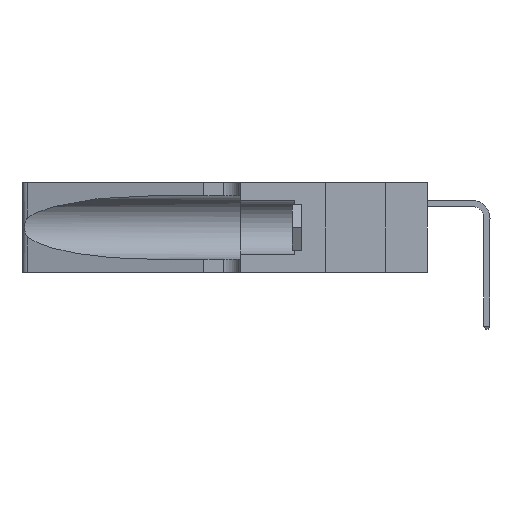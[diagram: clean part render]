
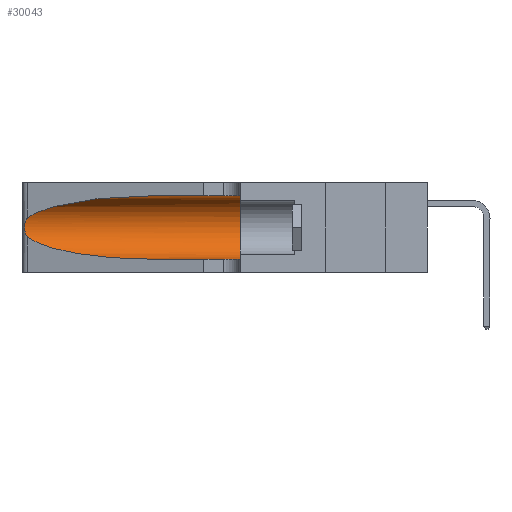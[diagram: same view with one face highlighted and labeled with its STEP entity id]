
A CAD part, left-side view. The second image highlights one B-rep face of the part: STEP entity #30043.
In plain terms, the highlighted cylindrical face has radius 3.308 mm (diameter 6.617 mm), a partial arc.
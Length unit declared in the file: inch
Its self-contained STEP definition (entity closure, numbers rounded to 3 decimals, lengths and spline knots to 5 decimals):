
#122 = VERTEX_POINT ( 'NONE', #33589 ) ;
#153 = EDGE_CURVE ( 'NONE', #27932, #27110, #19228, .T. ) ;
#482 = ORIENTED_EDGE ( 'NONE', *, *, #25769, .T. ) ;
#2545 = AXIS2_PLACEMENT_3D ( 'NONE', #18023, #11613, #39986 ) ;
#2652 = LINE ( 'NONE', #10013, #26861 ) ;
#4079 = CARTESIAN_POINT ( 'NONE',  ( 0.1305, 0.72297, 0.31525 ) ) ;
#4984 = CARTESIAN_POINT ( 'NONE',  ( 0.25787, 1.23484, 0.2124 ) ) ;
#6048 = CARTESIAN_POINT ( 'NONE',  ( 0.25487, 1.22718, 0.14631 ) ) ;
#6793 = CARTESIAN_POINT ( 'NONE',  ( 0.1305, 0.35, 0.05475 ) ) ;
#7227 = EDGE_CURVE ( 'NONE', #27932, #38747, #2652, .T. ) ;
#8102 = CARTESIAN_POINT ( 'NONE',  ( 0.26018, 1.23835, 0.19895 ) ) ;
#9229 = CARTESIAN_POINT ( 'NONE',  ( 0.2373, 1.15595, 0.08982 ) ) ;
#9741 = CYLINDRICAL_SURFACE ( 'NONE', #2545, 0.13025 ) ;
#10013 = CARTESIAN_POINT ( 'NONE',  ( 0.1305, 1.61858, 0.31525 ) ) ;
#11298 = CARTESIAN_POINT ( 'NONE',  ( 0.26075, 1.23896, 0.178 ) ) ;
#11610 = EDGE_CURVE ( 'NONE', #27110, #122, #30864, .T. ) ;
#11613 = DIRECTION ( 'NONE',  ( 0., -1., 0. ) ) ;
#11915 = CARTESIAN_POINT ( 'NONE',  ( 0.1305, 0.72297, 0.31525 ) ) ;
#12406 = CARTESIAN_POINT ( 'NONE',  ( 0.1305, 0.72297, 0.05475 ) ) ;
#13008 = VECTOR ( 'NONE', #24241, 39.37008 ) ;
#13343 = DIRECTION ( 'NONE',  ( 0., -1., 0. ) ) ;
#14002 = ORIENTED_EDGE ( 'NONE', *, *, #28887, .T. ) ;
#14014 = LINE ( 'NONE', #33591, #13008 ) ;
#14503 = CARTESIAN_POINT ( 'NONE',  ( 0.25856, 1.23593, 0.16098 ) ) ;
#15753 = VERTEX_POINT ( 'NONE', #29646 ) ;
#17562 = CARTESIAN_POINT ( 'NONE',  ( 0.25487, 1.22718, 0.22369 ) ) ;
#17705 = CARTESIAN_POINT ( 'NONE',  ( 0.25639, 1.23186, 0.15144 ) ) ;
#18023 = CARTESIAN_POINT ( 'NONE',  ( 0.1305, 1.61858, 0.185 ) ) ;
#18523 = DIRECTION ( 'NONE',  ( 0., 1., 0. ) ) ;
#19228 =( BOUNDED_CURVE ( )  B_SPLINE_CURVE ( 3, ( #11915, #34311, #33450, #20705 ),
 .UNSPECIFIED., .F., .F. ) 
 B_SPLINE_CURVE_WITH_KNOTS ( ( 4, 4 ),
 ( 1.5708, 2.84003 ),
 .UNSPECIFIED. ) 
 CURVE ( )  GEOMETRIC_REPRESENTATION_ITEM ( )  RATIONAL_B_SPLINE_CURVE ( ( 1., 0.87, 0.87, 1. ) ) 
 REPRESENTATION_ITEM ( '' )  );
#19772 = EDGE_CURVE ( 'NONE', #38747, #37189, #24844, .T. ) ;
#20705 = CARTESIAN_POINT ( 'NONE',  ( 0.25487, 1.22718, 0.22369 ) ) ;
#20757 = CARTESIAN_POINT ( 'NONE',  ( 0.25555, 1.22994, 0.2215 ) ) ;
#20896 = CARTESIAN_POINT ( 'NONE',  ( 0.25487, 1.22718, 0.14631 ) ) ;
#21916 = ORIENTED_EDGE ( 'NONE', *, *, #153, .T. ) ;
#22921 = ORIENTED_EDGE ( 'NONE', *, *, #11610, .T. ) ;
#23940 = CARTESIAN_POINT ( 'NONE',  ( 0.25639, 1.23184, 0.21858 ) ) ;
#24241 = DIRECTION ( 'NONE',  ( 0., -1., 0. ) ) ;
#24844 = CIRCLE ( 'NONE', #30788, 0.13025 ) ;
#25769 = EDGE_CURVE ( 'NONE', #15753, #37189, #14014, .T. ) ;
#26578 = FACE_OUTER_BOUND ( 'NONE', #40509, .T. ) ;
#26861 = VECTOR ( 'NONE', #13343, 39.37008 ) ;
#27091 = CARTESIAN_POINT ( 'NONE',  ( 0.25854, 1.2359, 0.20912 ) ) ;
#27110 = VERTEX_POINT ( 'NONE', #27984 ) ;
#27855 = CARTESIAN_POINT ( 'NONE',  ( 0.1305, 0.35, 0.31525 ) ) ;
#27932 = VERTEX_POINT ( 'NONE', #4079 ) ;
#27984 = CARTESIAN_POINT ( 'NONE',  ( 0.25487, 1.22718, 0.22369 ) ) ;
#28034 =( BOUNDED_CURVE ( )  B_SPLINE_CURVE ( 3, ( #6048, #9229, #31376, #12406 ),
 .UNSPECIFIED., .F., .F. ) 
 B_SPLINE_CURVE_WITH_KNOTS ( ( 4, 4 ),
 ( 3.44316, 4.71239 ),
 .UNSPECIFIED. ) 
 CURVE ( )  GEOMETRIC_REPRESENTATION_ITEM ( )  RATIONAL_B_SPLINE_CURVE ( ( 1., 0.87, 0.87, 1. ) ) 
 REPRESENTATION_ITEM ( '' )  );
#28653 = ORIENTED_EDGE ( 'NONE', *, *, #7227, .F. ) ;
#28887 = EDGE_CURVE ( 'NONE', #122, #15753, #28034, .T. ) ;
#29646 = CARTESIAN_POINT ( 'NONE',  ( 0.1305, 0.72297, 0.05475 ) ) ;
#30043 = ADVANCED_FACE ( 'NONE', ( #26578 ), #9741, .F. ) ;
#30272 = CARTESIAN_POINT ( 'NONE',  ( 0.26075, 1.23896, 0.19203 ) ) ;
#30788 = AXIS2_PLACEMENT_3D ( 'NONE', #37361, #18523, #40462 ) ;
#30864 = B_SPLINE_CURVE_WITH_KNOTS ( 'NONE', 3,
 ( #17562, #20757, #23940, #4984, #27091, #8102, #30272, #11298, #33427, #14503, #36586, #17705, #39670, #20896 ),
 .UNSPECIFIED., .F., .F.,
 ( 4, 2, 2, 2, 2, 2, 4 ),
 ( 0., 0.00027, 0.00053, 0.00107, 0.0016, 0.00187, 0.00214 ),
 .UNSPECIFIED. ) ;
#31376 = CARTESIAN_POINT ( 'NONE',  ( 0.18966, 0.96281, 0.05475 ) ) ;
#33427 = CARTESIAN_POINT ( 'NONE',  ( 0.26017, 1.23833, 0.17102 ) ) ;
#33450 = CARTESIAN_POINT ( 'NONE',  ( 0.2373, 1.15595, 0.28018 ) ) ;
#33589 = CARTESIAN_POINT ( 'NONE',  ( 0.25487, 1.22718, 0.14631 ) ) ;
#33591 = CARTESIAN_POINT ( 'NONE',  ( 0.1305, 1.61858, 0.05475 ) ) ;
#34299 = ORIENTED_EDGE ( 'NONE', *, *, #19772, .F. ) ;
#34311 = CARTESIAN_POINT ( 'NONE',  ( 0.18966, 0.96281, 0.31525 ) ) ;
#36586 = CARTESIAN_POINT ( 'NONE',  ( 0.25789, 1.23486, 0.15765 ) ) ;
#37189 = VERTEX_POINT ( 'NONE', #6793 ) ;
#37361 = CARTESIAN_POINT ( 'NONE',  ( 0.1305, 0.35, 0.185 ) ) ;
#38747 = VERTEX_POINT ( 'NONE', #27855 ) ;
#39670 = CARTESIAN_POINT ( 'NONE',  ( 0.25555, 1.22993, 0.14849 ) ) ;
#39986 = DIRECTION ( 'NONE',  ( 0., 0., -1. ) ) ;
#40462 = DIRECTION ( 'NONE',  ( 0., 0., 1. ) ) ;
#40509 = EDGE_LOOP ( 'NONE', ( #21916, #22921, #14002, #482, #34299, #28653 ) ) ;
